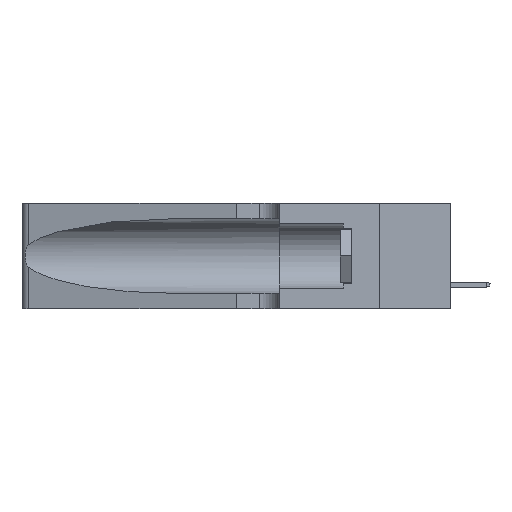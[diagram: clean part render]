
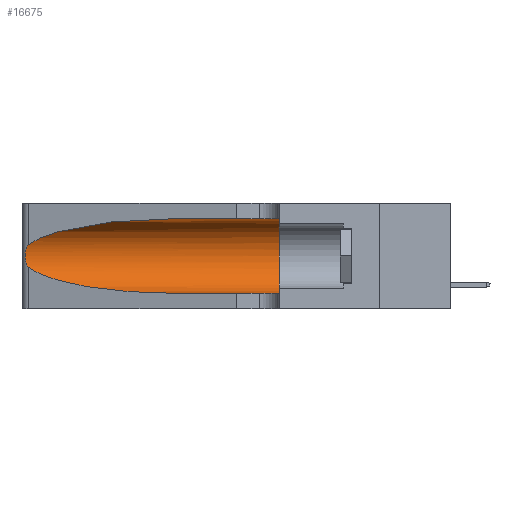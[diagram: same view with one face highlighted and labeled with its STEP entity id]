
A CAD part, left-side view. The second image highlights one B-rep face of the part: STEP entity #16675.
In plain terms, the highlighted cylindrical face has radius 3.308 mm (diameter 6.617 mm), a partial arc.
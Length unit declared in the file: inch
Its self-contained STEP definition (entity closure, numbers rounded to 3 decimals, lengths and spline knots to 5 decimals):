
#617 = LINE ( 'NONE', #38754, #38448 ) ;
#1230 = EDGE_CURVE ( 'NONE', #4211, #40032, #35283, .T. ) ;
#3485 = ORIENTED_EDGE ( 'NONE', *, *, #12775, .T. ) ;
#4211 = VERTEX_POINT ( 'NONE', #36412 ) ;
#4797 = CARTESIAN_POINT ( 'NONE',  ( 0.25639, 1.23186, 0.15144 ) ) ;
#5121 = EDGE_LOOP ( 'NONE', ( #3485, #22804, #13895, #37287, #17976, #13542 ) ) ;
#5138 = DIRECTION ( 'NONE',  ( 0., -1., 0. ) ) ;
#5433 = DIRECTION ( 'NONE',  ( 0., 0., 1. ) ) ;
#5561 = AXIS2_PLACEMENT_3D ( 'NONE', #36177, #15312, #5433 ) ;
#6936 = CARTESIAN_POINT ( 'NONE',  ( 0.25487, 1.22718, 0.22369 ) ) ;
#7102 = EDGE_CURVE ( 'NONE', #36795, #8674, #10884, .T. ) ;
#7727 = CARTESIAN_POINT ( 'NONE',  ( 0.25639, 1.23184, 0.21858 ) ) ;
#8674 = VERTEX_POINT ( 'NONE', #33325 ) ;
#9725 =( BOUNDED_CURVE ( )  B_SPLINE_CURVE ( 3, ( #31151, #20761, #14299, #6936 ),
 .UNSPECIFIED., .F., .F. ) 
 B_SPLINE_CURVE_WITH_KNOTS ( ( 4, 4 ),
 ( 1.5708, 2.84003 ),
 .UNSPECIFIED. ) 
 CURVE ( )  GEOMETRIC_REPRESENTATION_ITEM ( )  RATIONAL_B_SPLINE_CURVE ( ( 1., 0.87, 0.87, 1. ) ) 
 REPRESENTATION_ITEM ( '' )  );
#10276 = CARTESIAN_POINT ( 'NONE',  ( 0.2373, 1.15595, 0.08982 ) ) ;
#10884 = B_SPLINE_CURVE_WITH_KNOTS ( 'NONE', 3,
 ( #11756, #14670, #7727, #38459, #25239, #21868, #25014, #28149, #38680, #24578, #14887, #4797, #35344, #39133 ),
 .UNSPECIFIED., .F., .F.,
 ( 4, 2, 2, 2, 2, 2, 4 ),
 ( 0., 0.00027, 0.00053, 0.00107, 0.0016, 0.00187, 0.00214 ),
 .UNSPECIFIED. ) ;
#11756 = CARTESIAN_POINT ( 'NONE',  ( 0.25487, 1.22718, 0.22369 ) ) ;
#12102 = VERTEX_POINT ( 'NONE', #25180 ) ;
#12775 = EDGE_CURVE ( 'NONE', #4211, #36795, #9725, .T. ) ;
#13542 = ORIENTED_EDGE ( 'NONE', *, *, #1230, .F. ) ;
#13895 = ORIENTED_EDGE ( 'NONE', *, *, #18069, .T. ) ;
#14299 = CARTESIAN_POINT ( 'NONE',  ( 0.2373, 1.15595, 0.28018 ) ) ;
#14670 = CARTESIAN_POINT ( 'NONE',  ( 0.25555, 1.22994, 0.2215 ) ) ;
#14887 = CARTESIAN_POINT ( 'NONE',  ( 0.25789, 1.23486, 0.15765 ) ) ;
#15169 = EDGE_CURVE ( 'NONE', #40032, #12102, #29235, .T. ) ;
#15312 = DIRECTION ( 'NONE',  ( 0., 1., 0. ) ) ;
#16675 = ADVANCED_FACE ( 'NONE', ( #28928 ), #29377, .F. ) ;
#17461 = CARTESIAN_POINT ( 'NONE',  ( 0.18966, 0.96281, 0.05475 ) ) ;
#17976 = ORIENTED_EDGE ( 'NONE', *, *, #15169, .F. ) ;
#18069 = EDGE_CURVE ( 'NONE', #8674, #23763, #24025, .T. ) ;
#20761 = CARTESIAN_POINT ( 'NONE',  ( 0.18966, 0.96281, 0.31525 ) ) ;
#21820 = EDGE_CURVE ( 'NONE', #23763, #12102, #617, .T. ) ;
#21868 = CARTESIAN_POINT ( 'NONE',  ( 0.26018, 1.23835, 0.19895 ) ) ;
#22804 = ORIENTED_EDGE ( 'NONE', *, *, #7102, .T. ) ;
#23763 = VERTEX_POINT ( 'NONE', #39153 ) ;
#24025 =( BOUNDED_CURVE ( )  B_SPLINE_CURVE ( 3, ( #30500, #10276, #17461, #31155 ),
 .UNSPECIFIED., .F., .T. ) 
 B_SPLINE_CURVE_WITH_KNOTS ( ( 4, 4 ),
 ( 3.44316, 4.71239 ),
 .UNSPECIFIED. ) 
 CURVE ( )  GEOMETRIC_REPRESENTATION_ITEM ( )  RATIONAL_B_SPLINE_CURVE ( ( 1., 0.87, 0.87, 1. ) ) 
 REPRESENTATION_ITEM ( '' )  );
#24578 = CARTESIAN_POINT ( 'NONE',  ( 0.25856, 1.23593, 0.16098 ) ) ;
#25014 = CARTESIAN_POINT ( 'NONE',  ( 0.26075, 1.23896, 0.19203 ) ) ;
#25180 = CARTESIAN_POINT ( 'NONE',  ( 0.1305, 0.35, 0.05475 ) ) ;
#25239 = CARTESIAN_POINT ( 'NONE',  ( 0.25854, 1.2359, 0.20912 ) ) ;
#27009 = CARTESIAN_POINT ( 'NONE',  ( 0.1305, 0.35, 0.31525 ) ) ;
#27886 = AXIS2_PLACEMENT_3D ( 'NONE', #29593, #5138, #43285 ) ;
#28095 = DIRECTION ( 'NONE',  ( 0., -1., 0. ) ) ;
#28149 = CARTESIAN_POINT ( 'NONE',  ( 0.26075, 1.23896, 0.178 ) ) ;
#28928 = FACE_OUTER_BOUND ( 'NONE', #5121, .T. ) ;
#29235 = CIRCLE ( 'NONE', #5561, 0.13025 ) ;
#29377 = CYLINDRICAL_SURFACE ( 'NONE', #27886, 0.13025 ) ;
#29593 = CARTESIAN_POINT ( 'NONE',  ( 0.1305, 1.61858, 0.185 ) ) ;
#30500 = CARTESIAN_POINT ( 'NONE',  ( 0.25487, 1.22718, 0.14631 ) ) ;
#30605 = VECTOR ( 'NONE', #28095, 39.37008 ) ;
#31151 = CARTESIAN_POINT ( 'NONE',  ( 0.1305, 0.72297, 0.31525 ) ) ;
#31155 = CARTESIAN_POINT ( 'NONE',  ( 0.1305, 0.72297, 0.05475 ) ) ;
#31686 = CARTESIAN_POINT ( 'NONE',  ( 0.1305, 1.61858, 0.31525 ) ) ;
#33325 = CARTESIAN_POINT ( 'NONE',  ( 0.25487, 1.22718, 0.14631 ) ) ;
#35283 = LINE ( 'NONE', #31686, #30605 ) ;
#35344 = CARTESIAN_POINT ( 'NONE',  ( 0.25555, 1.22993, 0.14849 ) ) ;
#36177 = CARTESIAN_POINT ( 'NONE',  ( 0.1305, 0.35, 0.185 ) ) ;
#36412 = CARTESIAN_POINT ( 'NONE',  ( 0.1305, 0.72297, 0.31525 ) ) ;
#36795 = VERTEX_POINT ( 'NONE', #36965 ) ;
#36965 = CARTESIAN_POINT ( 'NONE',  ( 0.25487, 1.22718, 0.22369 ) ) ;
#37287 = ORIENTED_EDGE ( 'NONE', *, *, #21820, .T. ) ;
#38448 = VECTOR ( 'NONE', #41476, 39.37008 ) ;
#38459 = CARTESIAN_POINT ( 'NONE',  ( 0.25787, 1.23484, 0.2124 ) ) ;
#38680 = CARTESIAN_POINT ( 'NONE',  ( 0.26017, 1.23833, 0.17102 ) ) ;
#38754 = CARTESIAN_POINT ( 'NONE',  ( 0.1305, 1.61858, 0.05475 ) ) ;
#39133 = CARTESIAN_POINT ( 'NONE',  ( 0.25487, 1.22718, 0.14631 ) ) ;
#39153 = CARTESIAN_POINT ( 'NONE',  ( 0.1305, 0.72297, 0.05475 ) ) ;
#40032 = VERTEX_POINT ( 'NONE', #27009 ) ;
#41476 = DIRECTION ( 'NONE',  ( 0., -1., 0. ) ) ;
#43285 = DIRECTION ( 'NONE',  ( 0., 0., -1. ) ) ;
